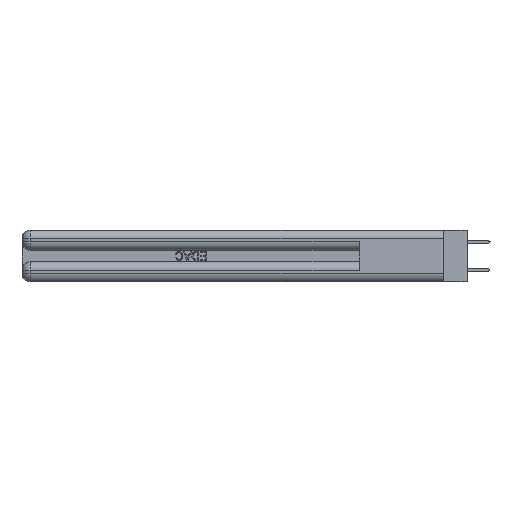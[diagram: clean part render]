
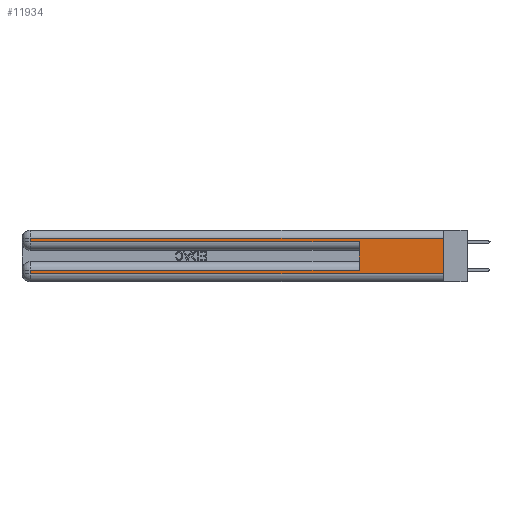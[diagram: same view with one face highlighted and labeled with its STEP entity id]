
A CAD part, left-side view. The second image highlights one B-rep face of the part: STEP entity #11934.
In plain terms, the highlighted planar face has unit normal (-1, 0, 0).
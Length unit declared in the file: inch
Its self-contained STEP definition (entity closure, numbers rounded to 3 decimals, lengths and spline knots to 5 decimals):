
#75 = ORIENTED_EDGE ( 'NONE', *, *, #19402, .T. ) ;
#476 = VECTOR ( 'NONE', #6381, 39.37008 ) ;
#887 = CARTESIAN_POINT ( 'NONE',  ( 0., 0., 0.06 ) ) ;
#967 = CARTESIAN_POINT ( 'NONE',  ( 0., 2.94, 0.37 ) ) ;
#1554 = EDGE_CURVE ( 'NONE', #46039, #18640, #6221, .T. ) ;
#1810 = VERTEX_POINT ( 'NONE', #8913 ) ;
#4333 = LINE ( 'NONE', #18377, #13071 ) ;
#4414 = VERTEX_POINT ( 'NONE', #31437 ) ;
#6221 = LINE ( 'NONE', #40254, #24691 ) ;
#6381 = DIRECTION ( 'NONE',  ( 0., 1., 0. ) ) ;
#6385 = CARTESIAN_POINT ( 'NONE',  ( 0., 0., 0.37 ) ) ;
#6832 = VERTEX_POINT ( 'NONE', #7139 ) ;
#7139 = CARTESIAN_POINT ( 'NONE',  ( 0., 2.94, 0.285 ) ) ;
#8194 = ORIENTED_EDGE ( 'NONE', *, *, #9714, .T. ) ;
#8420 = DIRECTION ( 'NONE',  ( 0., -1., 0. ) ) ;
#8505 = EDGE_CURVE ( 'NONE', #13604, #20659, #34345, .T. ) ;
#8913 = CARTESIAN_POINT ( 'NONE',  ( 0., 2.94, 0.06 ) ) ;
#9714 = EDGE_CURVE ( 'NONE', #18640, #6832, #4333, .T. ) ;
#10911 = LINE ( 'NONE', #42881, #12080 ) ;
#10918 = ORIENTED_EDGE ( 'NONE', *, *, #24181, .F. ) ;
#11604 = LINE ( 'NONE', #42984, #476 ) ;
#11934 = ADVANCED_FACE ( 'NONE', ( #15685 ), #14705, .F. ) ;
#12080 = VECTOR ( 'NONE', #21097, 39.37008 ) ;
#13071 = VECTOR ( 'NONE', #29399, 39.37008 ) ;
#13604 = VERTEX_POINT ( 'NONE', #31651 ) ;
#13766 = VECTOR ( 'NONE', #14455, 39.37008 ) ;
#14084 = ORIENTED_EDGE ( 'NONE', *, *, #1554, .T. ) ;
#14455 = DIRECTION ( 'NONE',  ( 0., 0., 1. ) ) ;
#14584 = LINE ( 'NONE', #6385, #41367 ) ;
#14705 = PLANE ( 'NONE',  #42496 ) ;
#15685 = FACE_OUTER_BOUND ( 'NONE', #41370, .T. ) ;
#16653 = ORIENTED_EDGE ( 'NONE', *, *, #8505, .F. ) ;
#18377 = CARTESIAN_POINT ( 'NONE',  ( 0., 2.94, 0.37 ) ) ;
#18398 = DIRECTION ( 'NONE',  ( 0., 0., -1. ) ) ;
#18426 = EDGE_CURVE ( 'NONE', #13604, #38985, #11604, .T. ) ;
#18640 = VERTEX_POINT ( 'NONE', #29527 ) ;
#19402 = EDGE_CURVE ( 'NONE', #1810, #4414, #46800, .T. ) ;
#19479 = DIRECTION ( 'NONE',  ( 0., 0., -1. ) ) ;
#20230 = LINE ( 'NONE', #967, #46904 ) ;
#20659 = VERTEX_POINT ( 'NONE', #22243 ) ;
#21097 = DIRECTION ( 'NONE',  ( 0., -1., 0. ) ) ;
#21824 = CARTESIAN_POINT ( 'NONE',  ( 0., 0.6, 0.145 ) ) ;
#22243 = CARTESIAN_POINT ( 'NONE',  ( 0., 0.6, 0.285 ) ) ;
#22314 = DIRECTION ( 'NONE',  ( 0., 1., 0. ) ) ;
#22512 = CARTESIAN_POINT ( 'NONE',  ( 0., 0., 0.31 ) ) ;
#24181 = EDGE_CURVE ( 'NONE', #46039, #4414, #14584, .T. ) ;
#24691 = VECTOR ( 'NONE', #22314, 39.37008 ) ;
#25919 = ORIENTED_EDGE ( 'NONE', *, *, #18426, .T. ) ;
#28584 = DIRECTION ( 'NONE',  ( 0., 0., -1. ) ) ;
#29205 = ORIENTED_EDGE ( 'NONE', *, *, #37298, .T. ) ;
#29399 = DIRECTION ( 'NONE',  ( 0., 0., -1. ) ) ;
#29527 = CARTESIAN_POINT ( 'NONE',  ( 0., 2.94, 0.31 ) ) ;
#30582 = ORIENTED_EDGE ( 'NONE', *, *, #35875, .T. ) ;
#31437 = CARTESIAN_POINT ( 'NONE',  ( 0., 0., 0.06 ) ) ;
#31651 = CARTESIAN_POINT ( 'NONE',  ( 0., 0.6, 0.085 ) ) ;
#32923 = CARTESIAN_POINT ( 'NONE',  ( 0., 0., 0.37 ) ) ;
#34345 = LINE ( 'NONE', #21824, #13766 ) ;
#35875 = EDGE_CURVE ( 'NONE', #38985, #1810, #20230, .T. ) ;
#37197 = VECTOR ( 'NONE', #8420, 39.37008 ) ;
#37298 = EDGE_CURVE ( 'NONE', #6832, #20659, #10911, .T. ) ;
#38985 = VERTEX_POINT ( 'NONE', #43683 ) ;
#40019 = DIRECTION ( 'NONE',  ( 1., 0., 0. ) ) ;
#40254 = CARTESIAN_POINT ( 'NONE',  ( 0., 0., 0.31 ) ) ;
#41367 = VECTOR ( 'NONE', #28584, 39.37008 ) ;
#41370 = EDGE_LOOP ( 'NONE', ( #10918, #14084, #8194, #29205, #16653, #25919, #30582, #75 ) ) ;
#42496 = AXIS2_PLACEMENT_3D ( 'NONE', #32923, #40019, #18398 ) ;
#42881 = CARTESIAN_POINT ( 'NONE',  ( 0., 0., 0.285 ) ) ;
#42984 = CARTESIAN_POINT ( 'NONE',  ( 0., 0., 0.085 ) ) ;
#43683 = CARTESIAN_POINT ( 'NONE',  ( 0., 2.94, 0.085 ) ) ;
#46039 = VERTEX_POINT ( 'NONE', #22512 ) ;
#46800 = LINE ( 'NONE', #887, #37197 ) ;
#46904 = VECTOR ( 'NONE', #19479, 39.37008 ) ;
